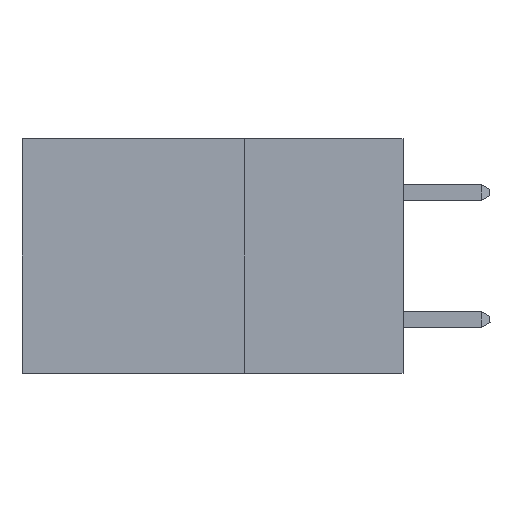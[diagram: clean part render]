
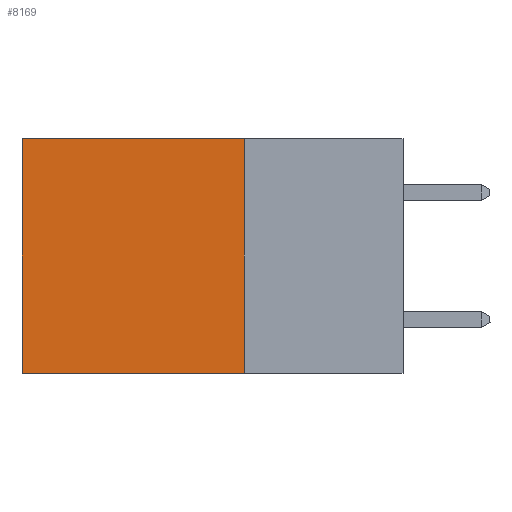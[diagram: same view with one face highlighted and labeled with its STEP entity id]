
A CAD part, left-side view. The second image highlights one B-rep face of the part: STEP entity #8169.
In plain terms, the highlighted planar face has unit normal (-1, 0, 0).
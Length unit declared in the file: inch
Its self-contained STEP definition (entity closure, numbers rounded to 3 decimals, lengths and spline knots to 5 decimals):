
#657 = VECTOR ( 'NONE', #11038, 39.37008 ) ;
#911 = FACE_OUTER_BOUND ( 'NONE', #4007, .T. ) ;
#918 = ORIENTED_EDGE ( 'NONE', *, *, #11342, .F. ) ;
#924 = CARTESIAN_POINT ( 'NONE',  ( 0.2875, 0.25, 0. ) ) ;
#1060 = EDGE_CURVE ( 'NONE', #1256, #10682, #8867, .T. ) ;
#1132 = CARTESIAN_POINT ( 'NONE',  ( 0.2875, 0.6, -0.37 ) ) ;
#1171 = DIRECTION ( 'NONE',  ( 0., 1., 0. ) ) ;
#1256 = VERTEX_POINT ( 'NONE', #13046 ) ;
#1383 = CARTESIAN_POINT ( 'NONE',  ( 0.2875, 0.25, -0.37 ) ) ;
#1600 = LINE ( 'NONE', #7330, #9749 ) ;
#2037 = DIRECTION ( 'NONE',  ( 0., 0., -1. ) ) ;
#2452 = DIRECTION ( 'NONE',  ( 0., 1., 0. ) ) ;
#2705 = CARTESIAN_POINT ( 'NONE',  ( 0.2875, 0.25, 0. ) ) ;
#3316 = ORIENTED_EDGE ( 'NONE', *, *, #3398, .T. ) ;
#3398 = EDGE_CURVE ( 'NONE', #6146, #1256, #9115, .T. ) ;
#3656 = VERTEX_POINT ( 'NONE', #1383 ) ;
#4007 = EDGE_LOOP ( 'NONE', ( #10722, #8918, #918, #3316 ) ) ;
#5391 = DIRECTION ( 'NONE',  ( 0., 0., -1. ) ) ;
#6146 = VERTEX_POINT ( 'NONE', #11628 ) ;
#6459 = VECTOR ( 'NONE', #2452, 39.37008 ) ;
#6826 = LINE ( 'NONE', #11437, #12531 ) ;
#7330 = CARTESIAN_POINT ( 'NONE',  ( 0.2875, 0.25, -0.37 ) ) ;
#7657 = EDGE_CURVE ( 'NONE', #3656, #10682, #1600, .T. ) ;
#8101 = DIRECTION ( 'NONE',  ( 1., 0., 0. ) ) ;
#8169 = ADVANCED_FACE ( 'NONE', ( #911 ), #12188, .F. ) ;
#8867 = LINE ( 'NONE', #10197, #657 ) ;
#8918 = ORIENTED_EDGE ( 'NONE', *, *, #7657, .F. ) ;
#9115 = LINE ( 'NONE', #2705, #6459 ) ;
#9749 = VECTOR ( 'NONE', #1171, 39.37008 ) ;
#10197 = CARTESIAN_POINT ( 'NONE',  ( 0.2875, 0.6, 0. ) ) ;
#10682 = VERTEX_POINT ( 'NONE', #1132 ) ;
#10722 = ORIENTED_EDGE ( 'NONE', *, *, #1060, .T. ) ;
#11038 = DIRECTION ( 'NONE',  ( 0., 0., -1. ) ) ;
#11342 = EDGE_CURVE ( 'NONE', #6146, #3656, #6826, .T. ) ;
#11430 = AXIS2_PLACEMENT_3D ( 'NONE', #924, #8101, #2037 ) ;
#11437 = CARTESIAN_POINT ( 'NONE',  ( 0.2875, 0.25, 0. ) ) ;
#11628 = CARTESIAN_POINT ( 'NONE',  ( 0.2875, 0.25, 0. ) ) ;
#12188 = PLANE ( 'NONE',  #11430 ) ;
#12531 = VECTOR ( 'NONE', #5391, 39.37008 ) ;
#13046 = CARTESIAN_POINT ( 'NONE',  ( 0.2875, 0.6, 0. ) ) ;
